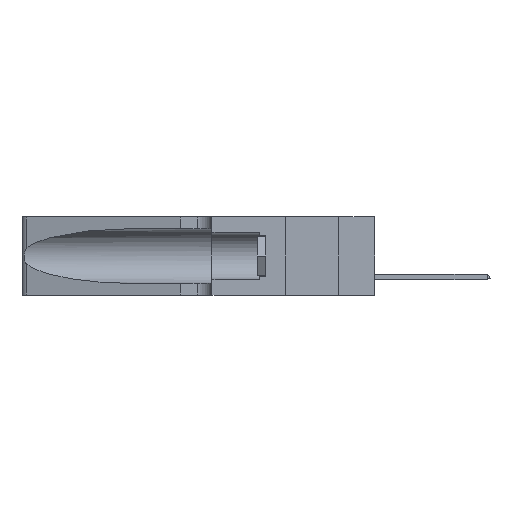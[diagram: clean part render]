
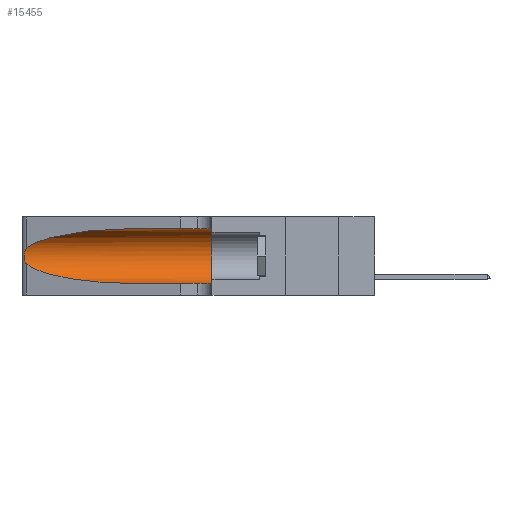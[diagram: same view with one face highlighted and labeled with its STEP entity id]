
A CAD part, left-side view. The second image highlights one B-rep face of the part: STEP entity #15455.
In plain terms, the highlighted cylindrical face has radius 3.308 mm (diameter 6.617 mm), a partial arc.
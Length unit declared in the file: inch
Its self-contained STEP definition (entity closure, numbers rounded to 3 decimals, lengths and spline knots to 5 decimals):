
#341 = CARTESIAN_POINT ( 'NONE',  ( 0.1305, 1.61858, 0.31525 ) ) ;
#773 = ORIENTED_EDGE ( 'NONE', *, *, #9962, .T. ) ;
#795 = EDGE_CURVE ( 'NONE', #25159, #25395, #15924, .T. ) ;
#926 = EDGE_CURVE ( 'NONE', #19395, #25159, #20811, .T. ) ;
#969 = ORIENTED_EDGE ( 'NONE', *, *, #795, .F. ) ;
#1552 = CARTESIAN_POINT ( 'NONE',  ( 0.26075, 1.23896, 0.19203 ) ) ;
#1757 = CARTESIAN_POINT ( 'NONE',  ( 0.25787, 1.23484, 0.2124 ) ) ;
#1860 = CARTESIAN_POINT ( 'NONE',  ( 0.25639, 1.23184, 0.21858 ) ) ;
#2649 = CARTESIAN_POINT ( 'NONE',  ( 0.1305, 0.35, 0.185 ) ) ;
#3467 = CARTESIAN_POINT ( 'NONE',  ( 0.25487, 1.22718, 0.22369 ) ) ;
#3938 = CARTESIAN_POINT ( 'NONE',  ( 0.25854, 1.2359, 0.20912 ) ) ;
#4357 = FACE_OUTER_BOUND ( 'NONE', #5620, .T. ) ;
#4733 = DIRECTION ( 'NONE',  ( 0., -1., 0. ) ) ;
#4955 = EDGE_CURVE ( 'NONE', #22367, #12115, #24104, .T. ) ;
#5098 = CARTESIAN_POINT ( 'NONE',  ( 0.25487, 1.22718, 0.22369 ) ) ;
#5546 = DIRECTION ( 'NONE',  ( 0., -1., 0. ) ) ;
#5620 = EDGE_LOOP ( 'NONE', ( #773, #19290, #28568, #10026, #969, #8449 ) ) ;
#6506 = CARTESIAN_POINT ( 'NONE',  ( 0.1305, 0.35, 0.05475 ) ) ;
#6756 =( BOUNDED_CURVE ( )  B_SPLINE_CURVE ( 3, ( #20114, #17953, #15405, #15797 ),
 .UNSPECIFIED., .F., .T. ) 
 B_SPLINE_CURVE_WITH_KNOTS ( ( 4, 4 ),
 ( 3.44316, 4.71239 ),
 .UNSPECIFIED. ) 
 CURVE ( )  GEOMETRIC_REPRESENTATION_ITEM ( )  RATIONAL_B_SPLINE_CURVE ( ( 1., 0.87, 0.87, 1. ) ) 
 REPRESENTATION_ITEM ( '' )  );
#7148 = CARTESIAN_POINT ( 'NONE',  ( 0.1305, 0.72297, 0.31525 ) ) ;
#7865 = CARTESIAN_POINT ( 'NONE',  ( 0.2373, 1.15595, 0.28018 ) ) ;
#7898 = AXIS2_PLACEMENT_3D ( 'NONE', #2649, #27298, #11722 ) ;
#8059 = EDGE_CURVE ( 'NONE', #26608, #25395, #10890, .T. ) ;
#8449 = ORIENTED_EDGE ( 'NONE', *, *, #926, .F. ) ;
#8526 = CARTESIAN_POINT ( 'NONE',  ( 0.26075, 1.23896, 0.178 ) ) ;
#8860 = CARTESIAN_POINT ( 'NONE',  ( 0.1305, 0.72297, 0.31525 ) ) ;
#8955 = CARTESIAN_POINT ( 'NONE',  ( 0.18966, 0.96281, 0.31525 ) ) ;
#9321 = EDGE_CURVE ( 'NONE', #12115, #26608, #6756, .T. ) ;
#9962 = EDGE_CURVE ( 'NONE', #19395, #22367, #15498, .T. ) ;
#10026 = ORIENTED_EDGE ( 'NONE', *, *, #8059, .T. ) ;
#10890 = LINE ( 'NONE', #13589, #22095 ) ;
#11722 = DIRECTION ( 'NONE',  ( 0., 0., 1. ) ) ;
#12115 = VERTEX_POINT ( 'NONE', #19187 ) ;
#12417 = CARTESIAN_POINT ( 'NONE',  ( 0.1305, 0.35, 0.31525 ) ) ;
#12709 = CARTESIAN_POINT ( 'NONE',  ( 0.26018, 1.23835, 0.19895 ) ) ;
#12904 = CARTESIAN_POINT ( 'NONE',  ( 0.25555, 1.22994, 0.2215 ) ) ;
#13589 = CARTESIAN_POINT ( 'NONE',  ( 0.1305, 1.61858, 0.05475 ) ) ;
#13897 = CARTESIAN_POINT ( 'NONE',  ( 0.1305, 1.61858, 0.185 ) ) ;
#14718 = CARTESIAN_POINT ( 'NONE',  ( 0.1305, 0.72297, 0.05475 ) ) ;
#15405 = CARTESIAN_POINT ( 'NONE',  ( 0.18966, 0.96281, 0.05475 ) ) ;
#15455 = ADVANCED_FACE ( 'NONE', ( #4357 ), #24288, .F. ) ;
#15498 =( BOUNDED_CURVE ( )  B_SPLINE_CURVE ( 3, ( #8860, #8955, #7865, #3467 ),
 .UNSPECIFIED., .F., .F. ) 
 B_SPLINE_CURVE_WITH_KNOTS ( ( 4, 4 ),
 ( 1.5708, 2.84003 ),
 .UNSPECIFIED. ) 
 CURVE ( )  GEOMETRIC_REPRESENTATION_ITEM ( )  RATIONAL_B_SPLINE_CURVE ( ( 1., 0.87, 0.87, 1. ) ) 
 REPRESENTATION_ITEM ( '' )  );
#15797 = CARTESIAN_POINT ( 'NONE',  ( 0.1305, 0.72297, 0.05475 ) ) ;
#15924 = CIRCLE ( 'NONE', #7898, 0.13025 ) ;
#16099 = DIRECTION ( 'NONE',  ( 0., -1., 0. ) ) ;
#17135 = CARTESIAN_POINT ( 'NONE',  ( 0.25487, 1.22718, 0.22369 ) ) ;
#17235 = CARTESIAN_POINT ( 'NONE',  ( 0.25856, 1.23593, 0.16098 ) ) ;
#17422 = CARTESIAN_POINT ( 'NONE',  ( 0.25639, 1.23186, 0.15144 ) ) ;
#17527 = CARTESIAN_POINT ( 'NONE',  ( 0.25555, 1.22993, 0.14849 ) ) ;
#17953 = CARTESIAN_POINT ( 'NONE',  ( 0.2373, 1.15595, 0.08982 ) ) ;
#19187 = CARTESIAN_POINT ( 'NONE',  ( 0.25487, 1.22718, 0.14631 ) ) ;
#19290 = ORIENTED_EDGE ( 'NONE', *, *, #4955, .T. ) ;
#19395 = VERTEX_POINT ( 'NONE', #7148 ) ;
#19467 = CARTESIAN_POINT ( 'NONE',  ( 0.25789, 1.23486, 0.15765 ) ) ;
#20114 = CARTESIAN_POINT ( 'NONE',  ( 0.25487, 1.22718, 0.14631 ) ) ;
#20811 = LINE ( 'NONE', #341, #25011 ) ;
#22095 = VECTOR ( 'NONE', #4733, 39.37008 ) ;
#22367 = VERTEX_POINT ( 'NONE', #5098 ) ;
#23025 = DIRECTION ( 'NONE',  ( 0., 0., -1. ) ) ;
#23487 = AXIS2_PLACEMENT_3D ( 'NONE', #13897, #5546, #23025 ) ;
#24104 = B_SPLINE_CURVE_WITH_KNOTS ( 'NONE', 3,
 ( #17135, #12904, #1860, #1757, #3938, #12709, #1552, #8526, #24167, #17235, #19467, #17422, #17527, #28473 ),
 .UNSPECIFIED., .F., .F.,
 ( 4, 2, 2, 2, 2, 2, 4 ),
 ( 0., 0.00027, 0.00053, 0.00107, 0.0016, 0.00187, 0.00214 ),
 .UNSPECIFIED. ) ;
#24167 = CARTESIAN_POINT ( 'NONE',  ( 0.26017, 1.23833, 0.17102 ) ) ;
#24288 = CYLINDRICAL_SURFACE ( 'NONE', #23487, 0.13025 ) ;
#25011 = VECTOR ( 'NONE', #16099, 39.37008 ) ;
#25159 = VERTEX_POINT ( 'NONE', #12417 ) ;
#25395 = VERTEX_POINT ( 'NONE', #6506 ) ;
#26608 = VERTEX_POINT ( 'NONE', #14718 ) ;
#27298 = DIRECTION ( 'NONE',  ( 0., 1., 0. ) ) ;
#28473 = CARTESIAN_POINT ( 'NONE',  ( 0.25487, 1.22718, 0.14631 ) ) ;
#28568 = ORIENTED_EDGE ( 'NONE', *, *, #9321, .T. ) ;
